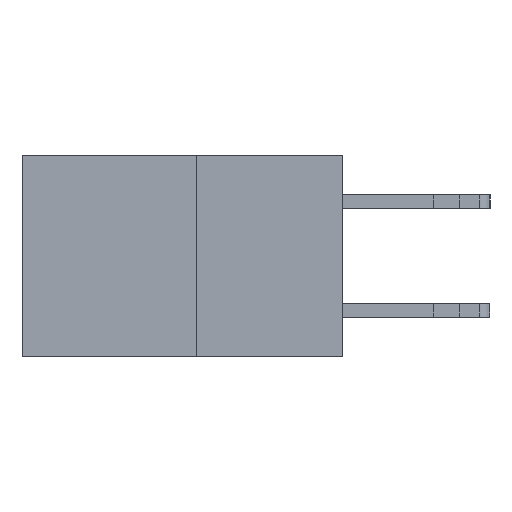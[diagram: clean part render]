
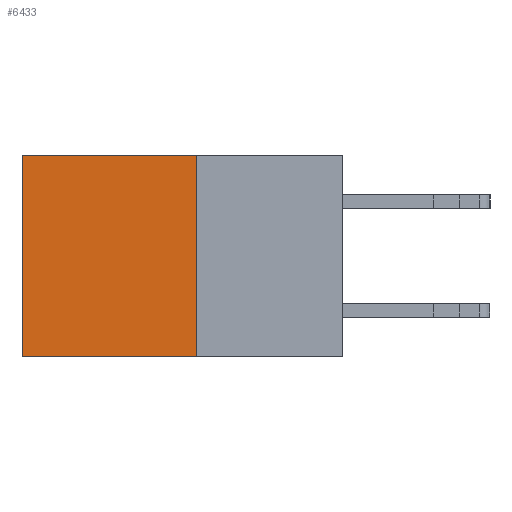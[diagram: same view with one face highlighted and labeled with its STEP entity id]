
A CAD part, left-side view. The second image highlights one B-rep face of the part: STEP entity #6433.
In plain terms, the highlighted planar face has unit normal (-1, 0, 0).
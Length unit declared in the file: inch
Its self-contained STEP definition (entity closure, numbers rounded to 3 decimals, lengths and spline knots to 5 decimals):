
#592 = LINE ( 'NONE', #10081, #8879 ) ;
#627 = ORIENTED_EDGE ( 'NONE', *, *, #9376, .T. ) ;
#1074 = LINE ( 'NONE', #5060, #6081 ) ;
#1752 = DIRECTION ( 'NONE',  ( 0., 0., -1. ) ) ;
#1925 = DIRECTION ( 'NONE',  ( 0., 1., 0. ) ) ;
#2667 = VECTOR ( 'NONE', #1752, 39.37008 ) ;
#2940 = EDGE_LOOP ( 'NONE', ( #627, #3604, #20560, #12822 ) ) ;
#3604 = ORIENTED_EDGE ( 'NONE', *, *, #10794, .F. ) ;
#4375 = VECTOR ( 'NONE', #7316, 39.37008 ) ;
#4916 = DIRECTION ( 'NONE',  ( 0., 0., -1. ) ) ;
#4969 = CARTESIAN_POINT ( 'NONE',  ( 0.277, 0.27, -0.37 ) ) ;
#5060 = CARTESIAN_POINT ( 'NONE',  ( 0.277, 0.27, 0. ) ) ;
#5085 = DIRECTION ( 'NONE',  ( 1., 0., 0. ) ) ;
#5215 = EDGE_CURVE ( 'NONE', #13267, #18004, #7727, .T. ) ;
#5611 = PLANE ( 'NONE',  #11866 ) ;
#6081 = VECTOR ( 'NONE', #14730, 39.37008 ) ;
#6338 = CARTESIAN_POINT ( 'NONE',  ( 0.277, 0.59, 0. ) ) ;
#6433 = ADVANCED_FACE ( 'NONE', ( #11665 ), #5611, .F. ) ;
#7137 = CARTESIAN_POINT ( 'NONE',  ( 0.277, 0.27, -0.37 ) ) ;
#7316 = DIRECTION ( 'NONE',  ( 0., 0., -1. ) ) ;
#7475 = VERTEX_POINT ( 'NONE', #6338 ) ;
#7727 = LINE ( 'NONE', #7137, #4375 ) ;
#8381 = CARTESIAN_POINT ( 'NONE',  ( 0.277, 0.59, -0.37 ) ) ;
#8879 = VECTOR ( 'NONE', #1925, 39.37008 ) ;
#9376 = EDGE_CURVE ( 'NONE', #7475, #13390, #20422, .T. ) ;
#10081 = CARTESIAN_POINT ( 'NONE',  ( 0.277, 0.27, -0.37 ) ) ;
#10794 = EDGE_CURVE ( 'NONE', #18004, #13390, #592, .T. ) ;
#11311 = CARTESIAN_POINT ( 'NONE',  ( 0.277, 0.27, 0. ) ) ;
#11665 = FACE_OUTER_BOUND ( 'NONE', #2940, .T. ) ;
#11866 = AXIS2_PLACEMENT_3D ( 'NONE', #4969, #5085, #4916 ) ;
#12822 = ORIENTED_EDGE ( 'NONE', *, *, #13404, .T. ) ;
#13267 = VERTEX_POINT ( 'NONE', #11311 ) ;
#13390 = VERTEX_POINT ( 'NONE', #21179 ) ;
#13404 = EDGE_CURVE ( 'NONE', #13267, #7475, #1074, .T. ) ;
#14730 = DIRECTION ( 'NONE',  ( 0., 1., 0. ) ) ;
#18004 = VERTEX_POINT ( 'NONE', #18398 ) ;
#18398 = CARTESIAN_POINT ( 'NONE',  ( 0.277, 0.27, -0.37 ) ) ;
#20422 = LINE ( 'NONE', #8381, #2667 ) ;
#20560 = ORIENTED_EDGE ( 'NONE', *, *, #5215, .F. ) ;
#21179 = CARTESIAN_POINT ( 'NONE',  ( 0.277, 0.59, -0.37 ) ) ;
